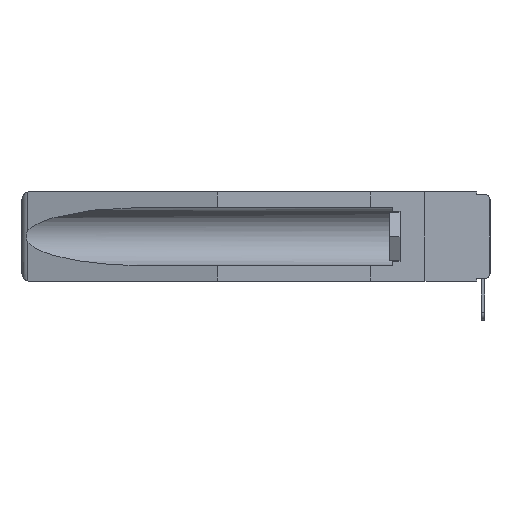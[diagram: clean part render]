
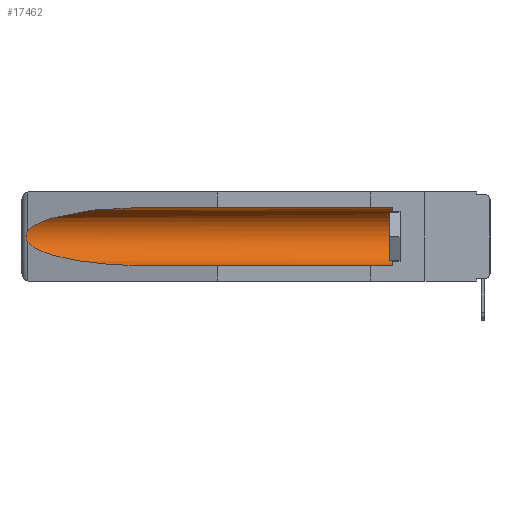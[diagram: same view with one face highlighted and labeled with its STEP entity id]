
A CAD part, left-side view. The second image highlights one B-rep face of the part: STEP entity #17462.
In plain terms, the highlighted cylindrical face has radius 2.857 mm (diameter 5.715 mm), a partial arc.
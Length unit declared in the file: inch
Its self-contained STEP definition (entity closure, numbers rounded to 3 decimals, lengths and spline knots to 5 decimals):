
#125 = VERTEX_POINT ( 'NONE', #12144 ) ;
#149 = DIRECTION ( 'NONE',  ( 0., 1., 0. ) ) ;
#227 = FACE_OUTER_BOUND ( 'NONE', #15991, .T. ) ;
#948 = CARTESIAN_POINT ( 'NONE',  ( 0.2675, 1.53308, -0.16763 ) ) ;
#1143 = ORIENTED_EDGE ( 'NONE', *, *, #9604, .F. ) ;
#1759 = CARTESIAN_POINT ( 'NONE',  ( 0.155, 1.07973, -0.059 ) ) ;
#1974 = CARTESIAN_POINT ( 'NONE',  ( 0.155, 0.126, -0.1715 ) ) ;
#2970 = CARTESIAN_POINT ( 'NONE',  ( 0.21114, 1.30732, -0.284 ) ) ;
#3897 = CARTESIAN_POINT ( 'NONE',  ( 0.155, -0.30754, -0.1715 ) ) ;
#3916 = EDGE_CURVE ( 'NONE', #125, #25875, #8728, .T. ) ;
#4516 = CIRCLE ( 'NONE', #5311, 0.1125 ) ;
#4632 =( BOUNDED_CURVE ( )  B_SPLINE_CURVE ( 3, ( #25954, #6567, #2970, #4808 ),
 .UNSPECIFIED., .F., .T. ) 
 B_SPLINE_CURVE_WITH_KNOTS ( ( 4, 4 ),
 ( 0.1948, 1.5708 ),
 .UNSPECIFIED. ) 
 CURVE ( )  GEOMETRIC_REPRESENTATION_ITEM ( )  RATIONAL_B_SPLINE_CURVE ( ( 1., 0.848, 0.848, 1. ) ) 
 REPRESENTATION_ITEM ( '' )  );
#4808 = CARTESIAN_POINT ( 'NONE',  ( 0.155, 1.07973, -0.284 ) ) ;
#5182 = CARTESIAN_POINT ( 'NONE',  ( 0.26654, 1.53092, -0.15636 ) ) ;
#5279 = CARTESIAN_POINT ( 'NONE',  ( 0.26655, 1.53094, -0.18657 ) ) ;
#5311 = AXIS2_PLACEMENT_3D ( 'NONE', #1974, #23240, #21333 ) ;
#5616 = ORIENTED_EDGE ( 'NONE', *, *, #3916, .T. ) ;
#5827 = DIRECTION ( 'NONE',  ( 0., 0., 1. ) ) ;
#6567 = CARTESIAN_POINT ( 'NONE',  ( 0.25451, 1.48313, -0.24835 ) ) ;
#7025 = CARTESIAN_POINT ( 'NONE',  ( 0.2675, 1.53308, -0.17534 ) ) ;
#7203 = CARTESIAN_POINT ( 'NONE',  ( 0.26537, 1.52718, -0.14972 ) ) ;
#8142 = VERTEX_POINT ( 'NONE', #1759 ) ;
#8159 = DIRECTION ( 'NONE',  ( 0., 1., 0. ) ) ;
#8545 = CARTESIAN_POINT ( 'NONE',  ( 0.155, 0.126, -0.284 ) ) ;
#8689 = CARTESIAN_POINT ( 'NONE',  ( 0.26537, 1.52718, -0.19328 ) ) ;
#8728 = B_SPLINE_CURVE_WITH_KNOTS ( 'NONE', 3,
 ( #7203, #9587, #5182, #26609, #948, #7025, #22017, #5279, #11457, #19950 ),
 .UNSPECIFIED., .F., .F.,
 ( 4, 2, 2, 2, 4 ),
 ( 0., 0.00029, 0.00058, 0.00087, 0.00117 ),
 .UNSPECIFIED. ) ;
#9587 = CARTESIAN_POINT ( 'NONE',  ( 0.26597, 1.52961, -0.15275 ) ) ;
#9604 = EDGE_CURVE ( 'NONE', #27254, #18143, #20264, .T. ) ;
#10864 = CYLINDRICAL_SURFACE ( 'NONE', #16407, 0.1125 ) ;
#11457 = CARTESIAN_POINT ( 'NONE',  ( 0.26597, 1.5296, -0.19026 ) ) ;
#12144 = CARTESIAN_POINT ( 'NONE',  ( 0.26537, 1.52718, -0.14972 ) ) ;
#12569 = EDGE_CURVE ( 'NONE', #25875, #18143, #4632, .T. ) ;
#12810 = CARTESIAN_POINT ( 'NONE',  ( 0.155, -0.30754, -0.284 ) ) ;
#13326 = EDGE_CURVE ( 'NONE', #14938, #8142, #19436, .T. ) ;
#13787 = ORIENTED_EDGE ( 'NONE', *, *, #12569, .T. ) ;
#14129 = ORIENTED_EDGE ( 'NONE', *, *, #25007, .T. ) ;
#14938 = VERTEX_POINT ( 'NONE', #27452 ) ;
#15991 = EDGE_LOOP ( 'NONE', ( #14129, #5616, #13787, #1143, #16807, #21055 ) ) ;
#16017 = CARTESIAN_POINT ( 'NONE',  ( 0.25451, 1.48313, -0.09465 ) ) ;
#16213 = CARTESIAN_POINT ( 'NONE',  ( 0.21114, 1.30732, -0.059 ) ) ;
#16407 = AXIS2_PLACEMENT_3D ( 'NONE', #3897, #8159, #5827 ) ;
#16807 = ORIENTED_EDGE ( 'NONE', *, *, #17535, .T. ) ;
#17462 = ADVANCED_FACE ( 'NONE', ( #227 ), #10864, .F. ) ;
#17535 = EDGE_CURVE ( 'NONE', #27254, #14938, #4516, .T. ) ;
#18143 = VERTEX_POINT ( 'NONE', #27140 ) ;
#18338 =( BOUNDED_CURVE ( )  B_SPLINE_CURVE ( 3, ( #20147, #16213, #16017, #22589 ),
 .UNSPECIFIED., .F., .F. ) 
 B_SPLINE_CURVE_WITH_KNOTS ( ( 4, 4 ),
 ( 4.71239, 6.08839 ),
 .UNSPECIFIED. ) 
 CURVE ( )  GEOMETRIC_REPRESENTATION_ITEM ( )  RATIONAL_B_SPLINE_CURVE ( ( 1., 0.848, 0.848, 1. ) ) 
 REPRESENTATION_ITEM ( '' )  );
#19436 = LINE ( 'NONE', #24719, #24882 ) ;
#19950 = CARTESIAN_POINT ( 'NONE',  ( 0.26537, 1.52718, -0.19328 ) ) ;
#20147 = CARTESIAN_POINT ( 'NONE',  ( 0.155, 1.07973, -0.059 ) ) ;
#20264 = LINE ( 'NONE', #12810, #21266 ) ;
#21055 = ORIENTED_EDGE ( 'NONE', *, *, #13326, .T. ) ;
#21266 = VECTOR ( 'NONE', #149, 39.37008 ) ;
#21333 = DIRECTION ( 'NONE',  ( 0., 0., 1. ) ) ;
#22017 = CARTESIAN_POINT ( 'NONE',  ( 0.2673, 1.53269, -0.17917 ) ) ;
#22589 = CARTESIAN_POINT ( 'NONE',  ( 0.26537, 1.52718, -0.14972 ) ) ;
#23240 = DIRECTION ( 'NONE',  ( 0., -1., 0. ) ) ;
#24719 = CARTESIAN_POINT ( 'NONE',  ( 0.155, -0.30754, -0.059 ) ) ;
#24882 = VECTOR ( 'NONE', #26969, 39.37008 ) ;
#25007 = EDGE_CURVE ( 'NONE', #8142, #125, #18338, .T. ) ;
#25875 = VERTEX_POINT ( 'NONE', #8689 ) ;
#25954 = CARTESIAN_POINT ( 'NONE',  ( 0.26537, 1.52718, -0.19328 ) ) ;
#26609 = CARTESIAN_POINT ( 'NONE',  ( 0.2673, 1.5327, -0.16383 ) ) ;
#26969 = DIRECTION ( 'NONE',  ( 0., 1., 0. ) ) ;
#27140 = CARTESIAN_POINT ( 'NONE',  ( 0.155, 1.07973, -0.284 ) ) ;
#27254 = VERTEX_POINT ( 'NONE', #8545 ) ;
#27452 = CARTESIAN_POINT ( 'NONE',  ( 0.155, 0.126, -0.059 ) ) ;
